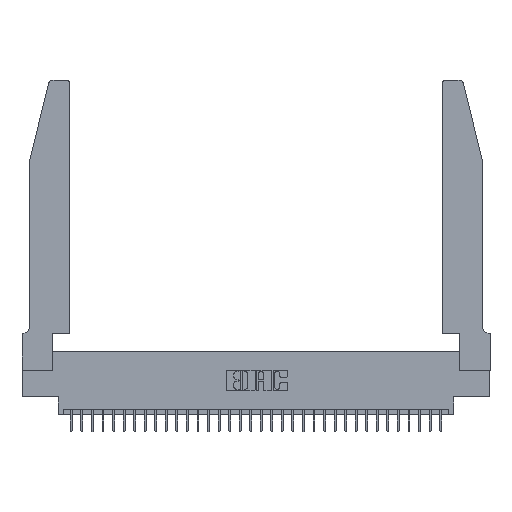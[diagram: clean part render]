
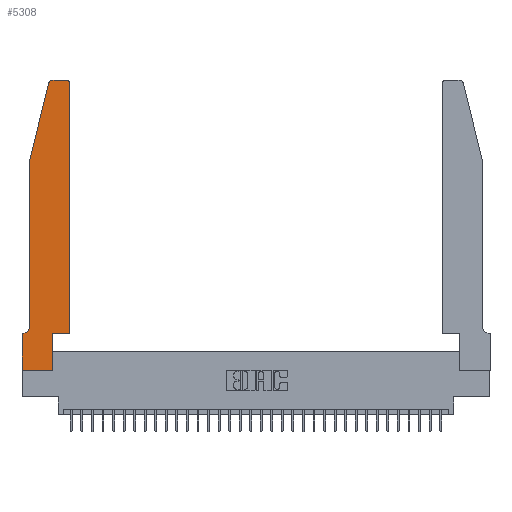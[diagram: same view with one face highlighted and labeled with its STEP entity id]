
A CAD part, top view. The second image highlights one B-rep face of the part: STEP entity #5308.
In plain terms, the highlighted planar face has unit normal (0, 0, 1).
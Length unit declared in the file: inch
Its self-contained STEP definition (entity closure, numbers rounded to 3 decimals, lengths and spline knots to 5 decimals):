
#314 = DIRECTION ( 'NONE',  ( 0., 0., 1. ) ) ;
#858 = CARTESIAN_POINT ( 'NONE',  ( 0., 0.35, 0.37 ) ) ;
#944 = CARTESIAN_POINT ( 'NONE',  ( 0.0055, 0.35, 0.37 ) ) ;
#1468 = LINE ( 'NONE', #9595, #33079 ) ;
#1747 = EDGE_CURVE ( 'NONE', #33806, #16211, #2248, .T. ) ;
#2217 = EDGE_CURVE ( 'NONE', #32795, #17285, #28245, .T. ) ;
#2248 = LINE ( 'NONE', #21932, #29063 ) ;
#2470 = VECTOR ( 'NONE', #32353, 39.37008 ) ;
#3019 = VERTEX_POINT ( 'NONE', #3360 ) ;
#3253 = DIRECTION ( 'NONE',  ( 0., 1., 0. ) ) ;
#3360 = CARTESIAN_POINT ( 'NONE',  ( 0.284, 2.75, 0.37 ) ) ;
#4612 = LINE ( 'NONE', #27782, #31666 ) ;
#5308 = ADVANCED_FACE ( 'NONE', ( #15244 ), #13520, .T. ) ;
#5343 = CARTESIAN_POINT ( 'NONE',  ( 0.4205, 2.72, 0.37 ) ) ;
#5725 = AXIS2_PLACEMENT_3D ( 'NONE', #15145, #33422, #17819 ) ;
#6347 = CIRCLE ( 'NONE', #22134, 0.03 ) ;
#6493 = LINE ( 'NONE', #7096, #18028 ) ;
#6842 = ORIENTED_EDGE ( 'NONE', *, *, #1747, .T. ) ;
#6932 = EDGE_CURVE ( 'NONE', #33376, #8342, #29528, .T. ) ;
#7096 = CARTESIAN_POINT ( 'NONE',  ( 0.0755, 2., 0.37 ) ) ;
#7108 = VECTOR ( 'NONE', #18031, 39.37008 ) ;
#7261 = CARTESIAN_POINT ( 'NONE',  ( 0.4505, 2.72, 0.37 ) ) ;
#7458 = CARTESIAN_POINT ( 'NONE',  ( 0., 0., 0.37 ) ) ;
#7500 = EDGE_CURVE ( 'NONE', #8342, #22303, #1468, .T. ) ;
#7993 = DIRECTION ( 'NONE',  ( 1., 0., 0. ) ) ;
#8342 = VERTEX_POINT ( 'NONE', #30204 ) ;
#9037 = EDGE_LOOP ( 'NONE', ( #27776, #28775, #14116, #6842, #28604, #25094, #22366, #33715, #19442, #19140, #33986, #22509 ) ) ;
#9357 = CARTESIAN_POINT ( 'NONE',  ( 0.0755, 0.42, 0.37 ) ) ;
#9595 = CARTESIAN_POINT ( 'NONE',  ( 0.2865, 0.35, 0.37 ) ) ;
#9712 = CARTESIAN_POINT ( 'NONE',  ( 0.284, 2.72, 0.37 ) ) ;
#9730 = DIRECTION ( 'NONE',  ( -0.239, -0.971, 0. ) ) ;
#9848 = CARTESIAN_POINT ( 'NONE',  ( 0.2865, 0.35, 0.37 ) ) ;
#10330 = LINE ( 'NONE', #16697, #2470 ) ;
#12218 = EDGE_CURVE ( 'NONE', #22303, #32795, #10330, .T. ) ;
#12381 = DIRECTION ( 'NONE',  ( 1., 0., 0. ) ) ;
#12882 = EDGE_CURVE ( 'NONE', #16211, #22009, #30785, .T. ) ;
#13520 = PLANE ( 'NONE',  #20332 ) ;
#14029 = EDGE_CURVE ( 'NONE', #17285, #23701, #25017, .T. ) ;
#14116 = ORIENTED_EDGE ( 'NONE', *, *, #23046, .T. ) ;
#15145 = CARTESIAN_POINT ( 'NONE',  ( 0.0055, 0.42, 0.37 ) ) ;
#15244 = FACE_OUTER_BOUND ( 'NONE', #9037, .T. ) ;
#15355 = CARTESIAN_POINT ( 'NONE',  ( 0.0755, 0.35, 0.37 ) ) ;
#16211 = VERTEX_POINT ( 'NONE', #9357 ) ;
#16518 = EDGE_CURVE ( 'NONE', #3019, #28251, #6347, .T. ) ;
#16697 = CARTESIAN_POINT ( 'NONE',  ( 0.4505, 0.35, 0.37 ) ) ;
#17188 = DIRECTION ( 'NONE',  ( 0., -1., 0. ) ) ;
#17231 = CARTESIAN_POINT ( 'NONE',  ( 0.2605, 2.75, 0.37 ) ) ;
#17285 = VERTEX_POINT ( 'NONE', #7261 ) ;
#17819 = DIRECTION ( 'NONE',  ( -1., 0., 0. ) ) ;
#18028 = VECTOR ( 'NONE', #9730, 39.37008 ) ;
#18031 = DIRECTION ( 'NONE',  ( -1., 0., 0. ) ) ;
#18418 = CARTESIAN_POINT ( 'NONE',  ( 0.4505, 0.35, 0.37 ) ) ;
#18846 = DIRECTION ( 'NONE',  ( 1., 0., 0. ) ) ;
#18929 = LINE ( 'NONE', #17231, #31975 ) ;
#19140 = ORIENTED_EDGE ( 'NONE', *, *, #12218, .T. ) ;
#19442 = ORIENTED_EDGE ( 'NONE', *, *, #7500, .T. ) ;
#19662 = AXIS2_PLACEMENT_3D ( 'NONE', #5343, #23764, #7993 ) ;
#19770 = CARTESIAN_POINT ( 'NONE',  ( 0., 0., 0.37 ) ) ;
#20332 = AXIS2_PLACEMENT_3D ( 'NONE', #31834, #314, #18846 ) ;
#21270 = VECTOR ( 'NONE', #34004, 39.37008 ) ;
#21876 = CARTESIAN_POINT ( 'NONE',  ( 0.4505, 0.35, 0.37 ) ) ;
#21932 = CARTESIAN_POINT ( 'NONE',  ( 0.0755, 2., 0.37 ) ) ;
#22009 = VERTEX_POINT ( 'NONE', #944 ) ;
#22134 = AXIS2_PLACEMENT_3D ( 'NONE', #9712, #28147, #12381 ) ;
#22139 = EDGE_CURVE ( 'NONE', #23701, #3019, #18929, .T. ) ;
#22303 = VERTEX_POINT ( 'NONE', #9848 ) ;
#22366 = ORIENTED_EDGE ( 'NONE', *, *, #33435, .T. ) ;
#22509 = ORIENTED_EDGE ( 'NONE', *, *, #14029, .T. ) ;
#22564 = DIRECTION ( 'NONE',  ( -1., 0., 0. ) ) ;
#23046 = EDGE_CURVE ( 'NONE', #28251, #33806, #6493, .T. ) ;
#23701 = VERTEX_POINT ( 'NONE', #30899 ) ;
#23764 = DIRECTION ( 'NONE',  ( 0., 0., 1. ) ) ;
#24533 = DIRECTION ( 'NONE',  ( 0., -1., 0. ) ) ;
#25017 = CIRCLE ( 'NONE', #19662, 0.03 ) ;
#25094 = ORIENTED_EDGE ( 'NONE', *, *, #27093, .T. ) ;
#25851 = DIRECTION ( 'NONE',  ( 1., 0., 0. ) ) ;
#27093 = EDGE_CURVE ( 'NONE', #22009, #33915, #28127, .T. ) ;
#27776 = ORIENTED_EDGE ( 'NONE', *, *, #22139, .T. ) ;
#27782 = CARTESIAN_POINT ( 'NONE',  ( 0., 0., 0.37 ) ) ;
#28127 = LINE ( 'NONE', #15355, #7108 ) ;
#28147 = DIRECTION ( 'NONE',  ( 0., 0., 1. ) ) ;
#28245 = LINE ( 'NONE', #18418, #21270 ) ;
#28251 = VERTEX_POINT ( 'NONE', #33174 ) ;
#28604 = ORIENTED_EDGE ( 'NONE', *, *, #12882, .T. ) ;
#28775 = ORIENTED_EDGE ( 'NONE', *, *, #16518, .T. ) ;
#29063 = VECTOR ( 'NONE', #24533, 39.37008 ) ;
#29221 = CARTESIAN_POINT ( 'NONE',  ( 0.0755, 2., 0.37 ) ) ;
#29528 = LINE ( 'NONE', #7458, #30326 ) ;
#30204 = CARTESIAN_POINT ( 'NONE',  ( 0.2865, 0., 0.37 ) ) ;
#30326 = VECTOR ( 'NONE', #25851, 39.37008 ) ;
#30785 = CIRCLE ( 'NONE', #5725, 0.07 ) ;
#30899 = CARTESIAN_POINT ( 'NONE',  ( 0.4205, 2.75, 0.37 ) ) ;
#31666 = VECTOR ( 'NONE', #17188, 39.37008 ) ;
#31834 = CARTESIAN_POINT ( 'NONE',  ( 0., 0.35, 0.37 ) ) ;
#31975 = VECTOR ( 'NONE', #22564, 39.37008 ) ;
#32353 = DIRECTION ( 'NONE',  ( 1., 0., 0. ) ) ;
#32795 = VERTEX_POINT ( 'NONE', #21876 ) ;
#33079 = VECTOR ( 'NONE', #3253, 39.37008 ) ;
#33174 = CARTESIAN_POINT ( 'NONE',  ( 0.25487, 2.72718, 0.37 ) ) ;
#33376 = VERTEX_POINT ( 'NONE', #19770 ) ;
#33422 = DIRECTION ( 'NONE',  ( 0., 0., -1. ) ) ;
#33435 = EDGE_CURVE ( 'NONE', #33915, #33376, #4612, .T. ) ;
#33715 = ORIENTED_EDGE ( 'NONE', *, *, #6932, .T. ) ;
#33806 = VERTEX_POINT ( 'NONE', #29221 ) ;
#33915 = VERTEX_POINT ( 'NONE', #858 ) ;
#33986 = ORIENTED_EDGE ( 'NONE', *, *, #2217, .T. ) ;
#34004 = DIRECTION ( 'NONE',  ( 0., 1., 0. ) ) ;
